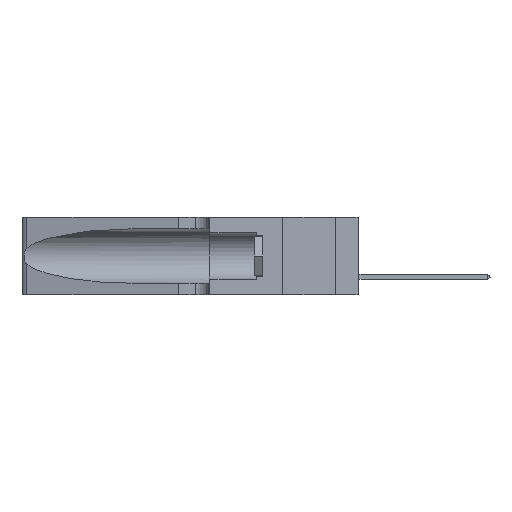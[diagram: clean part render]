
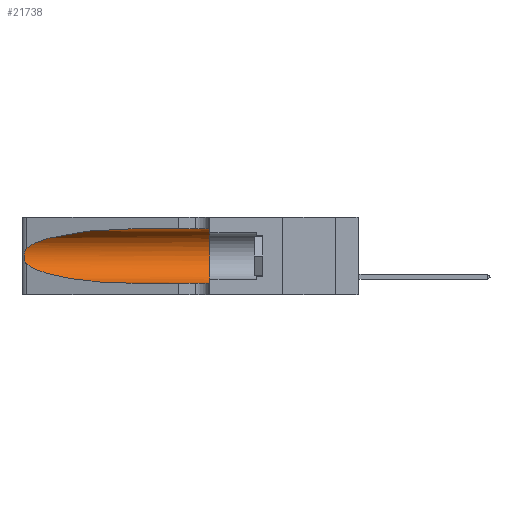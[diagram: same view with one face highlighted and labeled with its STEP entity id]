
A CAD part, left-side view. The second image highlights one B-rep face of the part: STEP entity #21738.
In plain terms, the highlighted cylindrical face has radius 3.308 mm (diameter 6.617 mm), a partial arc.
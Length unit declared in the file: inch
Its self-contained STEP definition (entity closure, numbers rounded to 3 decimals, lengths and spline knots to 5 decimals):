
#795 = EDGE_CURVE ( 'NONE', #18750, #20969, #16792, .T. ) ;
#1033 = CARTESIAN_POINT ( 'NONE',  ( 0.25639, 1.23184, 0.21858 ) ) ;
#1331 = CARTESIAN_POINT ( 'NONE',  ( 0.25487, 1.22718, 0.22369 ) ) ;
#1673 = DIRECTION ( 'NONE',  ( 0., 0., -1. ) ) ;
#3257 = VERTEX_POINT ( 'NONE', #27373 ) ;
#3361 = CARTESIAN_POINT ( 'NONE',  ( 0.25555, 1.22993, 0.14849 ) ) ;
#3466 = CARTESIAN_POINT ( 'NONE',  ( 0.25856, 1.23593, 0.16098 ) ) ;
#3769 = CARTESIAN_POINT ( 'NONE',  ( 0.26075, 1.23896, 0.178 ) ) ;
#4054 = ORIENTED_EDGE ( 'NONE', *, *, #795, .T. ) ;
#4969 = CARTESIAN_POINT ( 'NONE',  ( 0.25487, 1.22718, 0.22369 ) ) ;
#5076 = CARTESIAN_POINT ( 'NONE',  ( 0.2373, 1.15595, 0.28018 ) ) ;
#5513 = CARTESIAN_POINT ( 'NONE',  ( 0.1305, 0.35, 0.185 ) ) ;
#5798 = CARTESIAN_POINT ( 'NONE',  ( 0.25555, 1.22994, 0.2215 ) ) ;
#6079 = CARTESIAN_POINT ( 'NONE',  ( 0.26075, 1.23896, 0.19203 ) ) ;
#6292 = CARTESIAN_POINT ( 'NONE',  ( 0.1305, 0.72297, 0.05475 ) ) ;
#8040 = CARTESIAN_POINT ( 'NONE',  ( 0.25487, 1.22718, 0.14631 ) ) ;
#8197 = VECTOR ( 'NONE', #17718, 39.37008 ) ;
#8337 = CARTESIAN_POINT ( 'NONE',  ( 0.25789, 1.23486, 0.15765 ) ) ;
#10385 = CARTESIAN_POINT ( 'NONE',  ( 0.25787, 1.23484, 0.2124 ) ) ;
#10818 = CARTESIAN_POINT ( 'NONE',  ( 0.1305, 1.61858, 0.05475 ) ) ;
#10909 = CARTESIAN_POINT ( 'NONE',  ( 0.18966, 0.96281, 0.05475 ) ) ;
#11525 = B_SPLINE_CURVE_WITH_KNOTS ( 'NONE', 3,
 ( #1331, #5798, #1033, #10385, #15033, #17612, #6079, #3769, #22330, #3466, #8337, #29180, #3361, #8040 ),
 .UNSPECIFIED., .F., .F.,
 ( 4, 2, 2, 2, 2, 2, 4 ),
 ( 0., 0.00027, 0.00053, 0.00107, 0.0016, 0.00187, 0.00214 ),
 .UNSPECIFIED. ) ;
#11776 = ORIENTED_EDGE ( 'NONE', *, *, #13778, .F. ) ;
#11796 = CARTESIAN_POINT ( 'NONE',  ( 0.25487, 1.22718, 0.14631 ) ) ;
#11894 = VERTEX_POINT ( 'NONE', #19124 ) ;
#12529 = DIRECTION ( 'NONE',  ( 0., 0., 1. ) ) ;
#13149 = CARTESIAN_POINT ( 'NONE',  ( 0.2373, 1.15595, 0.08982 ) ) ;
#13778 = EDGE_CURVE ( 'NONE', #11894, #3257, #14479, .T. ) ;
#14235 = CARTESIAN_POINT ( 'NONE',  ( 0.18966, 0.96281, 0.31525 ) ) ;
#14479 = CIRCLE ( 'NONE', #23678, 0.13025 ) ;
#14815 = EDGE_CURVE ( 'NONE', #24804, #3257, #18077, .T. ) ;
#15033 = CARTESIAN_POINT ( 'NONE',  ( 0.25854, 1.2359, 0.20912 ) ) ;
#15091 = LINE ( 'NONE', #24947, #8197 ) ;
#15122 = VECTOR ( 'NONE', #25570, 39.37008 ) ;
#15306 = EDGE_CURVE ( 'NONE', #18750, #11894, #15091, .T. ) ;
#15331 = CARTESIAN_POINT ( 'NONE',  ( 0.25487, 1.22718, 0.22369 ) ) ;
#16178 = FACE_OUTER_BOUND ( 'NONE', #25390, .T. ) ;
#16792 =( BOUNDED_CURVE ( )  B_SPLINE_CURVE ( 3, ( #23532, #14235, #5076, #4969 ),
 .UNSPECIFIED., .F., .F. ) 
 B_SPLINE_CURVE_WITH_KNOTS ( ( 4, 4 ),
 ( 1.5708, 2.84003 ),
 .UNSPECIFIED. ) 
 CURVE ( )  GEOMETRIC_REPRESENTATION_ITEM ( )  RATIONAL_B_SPLINE_CURVE ( ( 1., 0.87, 0.87, 1. ) ) 
 REPRESENTATION_ITEM ( '' )  );
#17612 = CARTESIAN_POINT ( 'NONE',  ( 0.26018, 1.23835, 0.19895 ) ) ;
#17718 = DIRECTION ( 'NONE',  ( 0., -1., 0. ) ) ;
#18056 = DIRECTION ( 'NONE',  ( 0., -1., 0. ) ) ;
#18077 = LINE ( 'NONE', #10818, #15122 ) ;
#18750 = VERTEX_POINT ( 'NONE', #20065 ) ;
#19124 = CARTESIAN_POINT ( 'NONE',  ( 0.1305, 0.35, 0.31525 ) ) ;
#20065 = CARTESIAN_POINT ( 'NONE',  ( 0.1305, 0.72297, 0.31525 ) ) ;
#20317 = VERTEX_POINT ( 'NONE', #11796 ) ;
#20559 =( BOUNDED_CURVE ( )  B_SPLINE_CURVE ( 3, ( #27163, #13149, #10909, #25076 ),
 .UNSPECIFIED., .F., .F. ) 
 B_SPLINE_CURVE_WITH_KNOTS ( ( 4, 4 ),
 ( 3.44316, 4.71239 ),
 .UNSPECIFIED. ) 
 CURVE ( )  GEOMETRIC_REPRESENTATION_ITEM ( )  RATIONAL_B_SPLINE_CURVE ( ( 1., 0.87, 0.87, 1. ) ) 
 REPRESENTATION_ITEM ( '' )  );
#20969 = VERTEX_POINT ( 'NONE', #15331 ) ;
#21738 = ADVANCED_FACE ( 'NONE', ( #16178 ), #27532, .F. ) ;
#22091 = AXIS2_PLACEMENT_3D ( 'NONE', #29899, #18056, #1673 ) ;
#22330 = CARTESIAN_POINT ( 'NONE',  ( 0.26017, 1.23833, 0.17102 ) ) ;
#23215 = ORIENTED_EDGE ( 'NONE', *, *, #15306, .F. ) ;
#23498 = ORIENTED_EDGE ( 'NONE', *, *, #14815, .T. ) ;
#23532 = CARTESIAN_POINT ( 'NONE',  ( 0.1305, 0.72297, 0.31525 ) ) ;
#23678 = AXIS2_PLACEMENT_3D ( 'NONE', #5513, #23854, #12529 ) ;
#23854 = DIRECTION ( 'NONE',  ( 0., 1., 0. ) ) ;
#24804 = VERTEX_POINT ( 'NONE', #6292 ) ;
#24947 = CARTESIAN_POINT ( 'NONE',  ( 0.1305, 1.61858, 0.31525 ) ) ;
#25076 = CARTESIAN_POINT ( 'NONE',  ( 0.1305, 0.72297, 0.05475 ) ) ;
#25108 = ORIENTED_EDGE ( 'NONE', *, *, #29689, .T. ) ;
#25390 = EDGE_LOOP ( 'NONE', ( #4054, #27754, #25108, #23498, #11776, #23215 ) ) ;
#25570 = DIRECTION ( 'NONE',  ( 0., -1., 0. ) ) ;
#26584 = EDGE_CURVE ( 'NONE', #20969, #20317, #11525, .T. ) ;
#27163 = CARTESIAN_POINT ( 'NONE',  ( 0.25487, 1.22718, 0.14631 ) ) ;
#27373 = CARTESIAN_POINT ( 'NONE',  ( 0.1305, 0.35, 0.05475 ) ) ;
#27532 = CYLINDRICAL_SURFACE ( 'NONE', #22091, 0.13025 ) ;
#27754 = ORIENTED_EDGE ( 'NONE', *, *, #26584, .T. ) ;
#29180 = CARTESIAN_POINT ( 'NONE',  ( 0.25639, 1.23186, 0.15144 ) ) ;
#29689 = EDGE_CURVE ( 'NONE', #20317, #24804, #20559, .T. ) ;
#29899 = CARTESIAN_POINT ( 'NONE',  ( 0.1305, 1.61858, 0.185 ) ) ;
